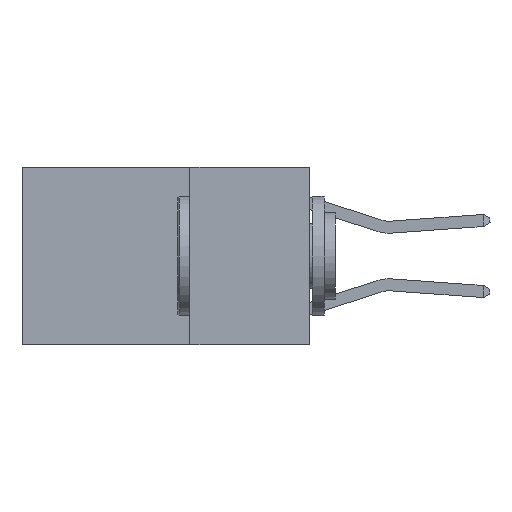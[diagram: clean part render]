
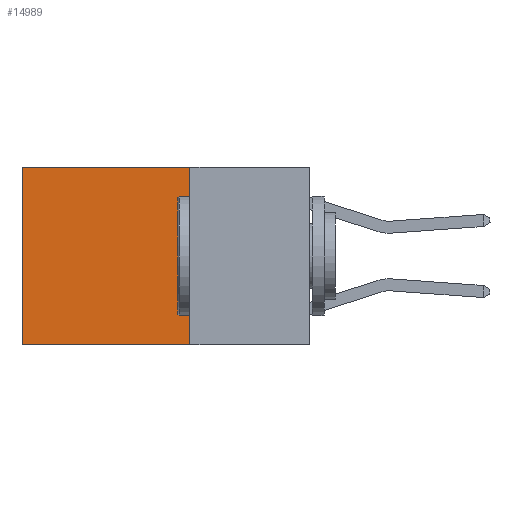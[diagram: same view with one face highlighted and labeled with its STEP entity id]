
A CAD part, left-side view. The second image highlights one B-rep face of the part: STEP entity #14989.
In plain terms, the highlighted planar face has unit normal (-1, 0, 0).
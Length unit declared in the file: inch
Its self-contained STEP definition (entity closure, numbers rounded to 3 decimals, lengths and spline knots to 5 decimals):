
#323 = CARTESIAN_POINT ( 'NONE',  ( 0.2625, 0.25, 0. ) ) ;
#1184 = CARTESIAN_POINT ( 'NONE',  ( 0.2625, 0.6, 0. ) ) ;
#1376 = EDGE_CURVE ( 'NONE', #16489, #8048, #23394, .T. ) ;
#2081 = VECTOR ( 'NONE', #16767, 39.37008 ) ;
#2302 = CARTESIAN_POINT ( 'NONE',  ( 0.2625, 0.6, 0. ) ) ;
#3323 = DIRECTION ( 'NONE',  ( 0., 0., -1. ) ) ;
#3646 = VECTOR ( 'NONE', #6378, 39.37008 ) ;
#4990 = EDGE_CURVE ( 'NONE', #13503, #24650, #23024, .T. ) ;
#6002 = DIRECTION ( 'NONE',  ( 0., 1., 0. ) ) ;
#6378 = DIRECTION ( 'NONE',  ( 0., 1., 0. ) ) ;
#6507 = EDGE_CURVE ( 'NONE', #13503, #16489, #17777, .T. ) ;
#7635 = CARTESIAN_POINT ( 'NONE',  ( 0.2625, 0.25, -0.37 ) ) ;
#8048 = VERTEX_POINT ( 'NONE', #19517 ) ;
#11731 = ORIENTED_EDGE ( 'NONE', *, *, #1376, .F. ) ;
#13503 = VERTEX_POINT ( 'NONE', #19715 ) ;
#14363 = ORIENTED_EDGE ( 'NONE', *, *, #4990, .T. ) ;
#14830 = LINE ( 'NONE', #2302, #2081 ) ;
#14989 = ADVANCED_FACE ( 'NONE', ( #30363 ), #30036, .F. ) ;
#15304 = AXIS2_PLACEMENT_3D ( 'NONE', #323, #20228, #25379 ) ;
#16489 = VERTEX_POINT ( 'NONE', #7635 ) ;
#16767 = DIRECTION ( 'NONE',  ( 0., 0., -1. ) ) ;
#17509 = VECTOR ( 'NONE', #3323, 39.37008 ) ;
#17777 = LINE ( 'NONE', #22910, #17509 ) ;
#18383 = ORIENTED_EDGE ( 'NONE', *, *, #6507, .F. ) ;
#18585 = ORIENTED_EDGE ( 'NONE', *, *, #20120, .T. ) ;
#19517 = CARTESIAN_POINT ( 'NONE',  ( 0.2625, 0.6, -0.37 ) ) ;
#19715 = CARTESIAN_POINT ( 'NONE',  ( 0.2625, 0.25, 0. ) ) ;
#20120 = EDGE_CURVE ( 'NONE', #24650, #8048, #14830, .T. ) ;
#20228 = DIRECTION ( 'NONE',  ( 1., 0., 0. ) ) ;
#22910 = CARTESIAN_POINT ( 'NONE',  ( 0.2625, 0.25, 0. ) ) ;
#23024 = LINE ( 'NONE', #23343, #25975 ) ;
#23343 = CARTESIAN_POINT ( 'NONE',  ( 0.2625, 0.25, 0. ) ) ;
#23394 = LINE ( 'NONE', #26290, #3646 ) ;
#24650 = VERTEX_POINT ( 'NONE', #1184 ) ;
#25379 = DIRECTION ( 'NONE',  ( 0., 0., -1. ) ) ;
#25975 = VECTOR ( 'NONE', #6002, 39.37008 ) ;
#26290 = CARTESIAN_POINT ( 'NONE',  ( 0.2625, 0.25, -0.37 ) ) ;
#27691 = EDGE_LOOP ( 'NONE', ( #18585, #11731, #18383, #14363 ) ) ;
#30036 = PLANE ( 'NONE',  #15304 ) ;
#30363 = FACE_OUTER_BOUND ( 'NONE', #27691, .T. ) ;
